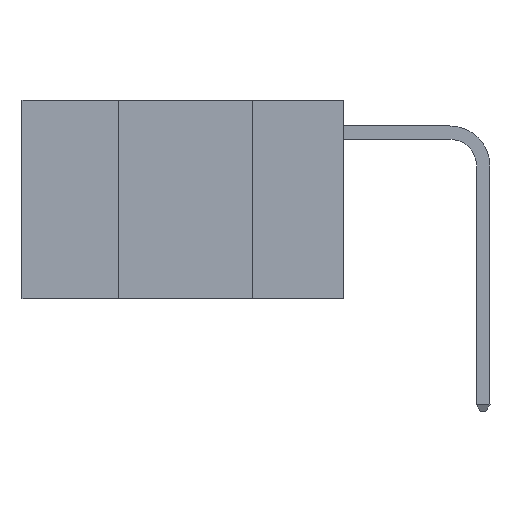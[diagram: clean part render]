
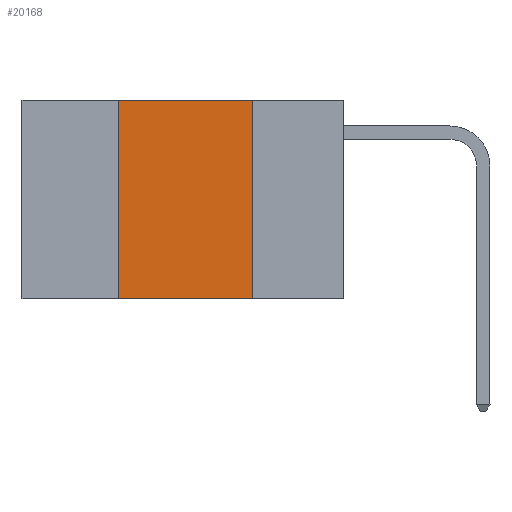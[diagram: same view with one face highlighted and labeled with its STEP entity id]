
A CAD part, left-side view. The second image highlights one B-rep face of the part: STEP entity #20168.
In plain terms, the highlighted planar face has unit normal (-1, 0, 0).
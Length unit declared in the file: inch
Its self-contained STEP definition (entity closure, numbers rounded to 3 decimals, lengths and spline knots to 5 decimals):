
#219 = VERTEX_POINT ( 'NONE', #18024 ) ;
#487 = CARTESIAN_POINT ( 'NONE',  ( 0., 0.17, 0. ) ) ;
#1770 = EDGE_CURVE ( 'NONE', #2372, #14694, #5748, .T. ) ;
#2372 = VERTEX_POINT ( 'NONE', #6132 ) ;
#3268 = DIRECTION ( 'NONE',  ( 0., 0., -1. ) ) ;
#4617 = EDGE_LOOP ( 'NONE', ( #8446, #12694, #19048, #5040 ) ) ;
#5040 = ORIENTED_EDGE ( 'NONE', *, *, #8198, .T. ) ;
#5748 = LINE ( 'NONE', #20206, #18364 ) ;
#5787 = VERTEX_POINT ( 'NONE', #15102 ) ;
#6132 = CARTESIAN_POINT ( 'NONE',  ( 0., 0.42, -0.37 ) ) ;
#6358 = DIRECTION ( 'NONE',  ( 0., 0., -1. ) ) ;
#8124 = CARTESIAN_POINT ( 'NONE',  ( 0., 0.6, 0. ) ) ;
#8198 = EDGE_CURVE ( 'NONE', #2372, #5787, #17450, .T. ) ;
#8446 = ORIENTED_EDGE ( 'NONE', *, *, #17462, .F. ) ;
#8896 = DIRECTION ( 'NONE',  ( 0., -1., 0. ) ) ;
#9407 = AXIS2_PLACEMENT_3D ( 'NONE', #8124, #19275, #3268 ) ;
#12313 = CARTESIAN_POINT ( 'NONE',  ( 0., 0.6, 0. ) ) ;
#12639 = VECTOR ( 'NONE', #8896, 39.37008 ) ;
#12694 = ORIENTED_EDGE ( 'NONE', *, *, #18228, .F. ) ;
#13795 = DIRECTION ( 'NONE',  ( 0., 0., 1. ) ) ;
#13918 = VECTOR ( 'NONE', #6358, 39.37008 ) ;
#14059 = CARTESIAN_POINT ( 'NONE',  ( 0., 0.42, 0. ) ) ;
#14315 = PLANE ( 'NONE',  #9407 ) ;
#14512 = LINE ( 'NONE', #487, #13918 ) ;
#14694 = VERTEX_POINT ( 'NONE', #14059 ) ;
#15102 = CARTESIAN_POINT ( 'NONE',  ( 0., 0.17, -0.37 ) ) ;
#15924 = DIRECTION ( 'NONE',  ( 0., -1., 0. ) ) ;
#17450 = LINE ( 'NONE', #17563, #17554 ) ;
#17462 = EDGE_CURVE ( 'NONE', #219, #5787, #14512, .T. ) ;
#17554 = VECTOR ( 'NONE', #15924, 39.37008 ) ;
#17563 = CARTESIAN_POINT ( 'NONE',  ( 0., 0.6, -0.37 ) ) ;
#18024 = CARTESIAN_POINT ( 'NONE',  ( 0., 0.17, 0. ) ) ;
#18228 = EDGE_CURVE ( 'NONE', #14694, #219, #20260, .T. ) ;
#18364 = VECTOR ( 'NONE', #13795, 39.37008 ) ;
#18746 = FACE_OUTER_BOUND ( 'NONE', #4617, .T. ) ;
#19048 = ORIENTED_EDGE ( 'NONE', *, *, #1770, .F. ) ;
#19275 = DIRECTION ( 'NONE',  ( 1., 0., 0. ) ) ;
#20168 = ADVANCED_FACE ( 'NONE', ( #18746 ), #14315, .F. ) ;
#20206 = CARTESIAN_POINT ( 'NONE',  ( 0., 0.42, 0. ) ) ;
#20260 = LINE ( 'NONE', #12313, #12639 ) ;
